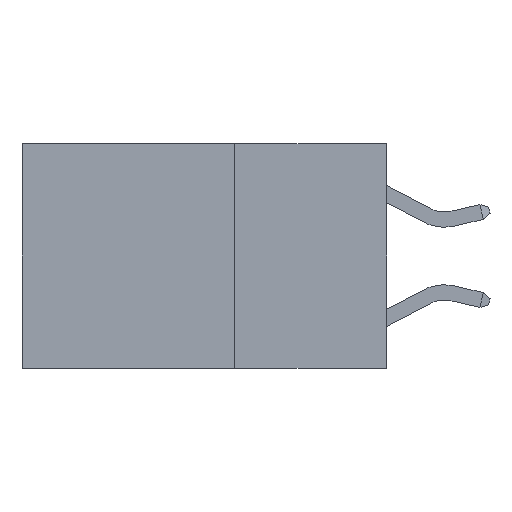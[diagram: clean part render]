
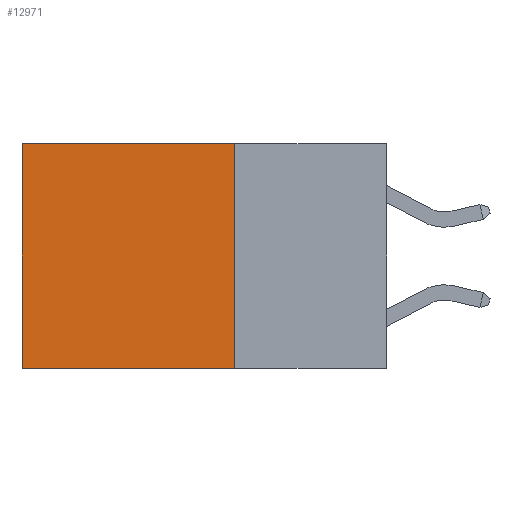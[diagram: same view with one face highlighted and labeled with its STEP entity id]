
A CAD part, left-side view. The second image highlights one B-rep face of the part: STEP entity #12971.
In plain terms, the highlighted planar face has unit normal (-1, 0, 0).
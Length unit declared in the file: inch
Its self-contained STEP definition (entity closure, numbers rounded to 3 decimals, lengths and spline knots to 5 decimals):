
#107 = VERTEX_POINT ( 'NONE', #5444 ) ;
#319 = PLANE ( 'NONE',  #3180 ) ;
#429 = CARTESIAN_POINT ( 'NONE',  ( 0.2625, 0.25, 0. ) ) ;
#506 = LINE ( 'NONE', #429, #14745 ) ;
#644 = DIRECTION ( 'NONE',  ( 0., 0., -1. ) ) ;
#1274 = VECTOR ( 'NONE', #12348, 39.37008 ) ;
#1816 = CARTESIAN_POINT ( 'NONE',  ( 0.2625, 0.6, -0.37 ) ) ;
#1836 = DIRECTION ( 'NONE',  ( 0., 0., -1. ) ) ;
#2252 = EDGE_LOOP ( 'NONE', ( #14381, #6729, #11589, #6524 ) ) ;
#3171 = EDGE_CURVE ( 'NONE', #15332, #3695, #506, .T. ) ;
#3180 = AXIS2_PLACEMENT_3D ( 'NONE', #10786, #8095, #644 ) ;
#3695 = VERTEX_POINT ( 'NONE', #15940 ) ;
#4331 = VECTOR ( 'NONE', #13352, 39.37008 ) ;
#5444 = CARTESIAN_POINT ( 'NONE',  ( 0.2625, 0.25, -0.37 ) ) ;
#5602 = VECTOR ( 'NONE', #1836, 39.37008 ) ;
#5854 = CARTESIAN_POINT ( 'NONE',  ( 0.2625, 0.25, -0.37 ) ) ;
#6524 = ORIENTED_EDGE ( 'NONE', *, *, #3171, .T. ) ;
#6729 = ORIENTED_EDGE ( 'NONE', *, *, #10629, .F. ) ;
#7406 = CARTESIAN_POINT ( 'NONE',  ( 0.2625, 0.6, 0. ) ) ;
#8095 = DIRECTION ( 'NONE',  ( 1., 0., 0. ) ) ;
#9372 = LINE ( 'NONE', #10867, #5602 ) ;
#10629 = EDGE_CURVE ( 'NONE', #107, #14761, #12261, .T. ) ;
#10786 = CARTESIAN_POINT ( 'NONE',  ( 0.2625, 0.25, 0. ) ) ;
#10867 = CARTESIAN_POINT ( 'NONE',  ( 0.2625, 0.25, 0. ) ) ;
#11589 = ORIENTED_EDGE ( 'NONE', *, *, #12950, .F. ) ;
#12261 = LINE ( 'NONE', #5854, #1274 ) ;
#12348 = DIRECTION ( 'NONE',  ( 0., 1., 0. ) ) ;
#12950 = EDGE_CURVE ( 'NONE', #15332, #107, #9372, .T. ) ;
#12971 = ADVANCED_FACE ( 'NONE', ( #13560 ), #319, .F. ) ;
#13352 = DIRECTION ( 'NONE',  ( 0., 0., -1. ) ) ;
#13560 = FACE_OUTER_BOUND ( 'NONE', #2252, .T. ) ;
#13649 = LINE ( 'NONE', #7406, #4331 ) ;
#14381 = ORIENTED_EDGE ( 'NONE', *, *, #15922, .T. ) ;
#14436 = DIRECTION ( 'NONE',  ( 0., 1., 0. ) ) ;
#14745 = VECTOR ( 'NONE', #14436, 39.37008 ) ;
#14761 = VERTEX_POINT ( 'NONE', #1816 ) ;
#15332 = VERTEX_POINT ( 'NONE', #16239 ) ;
#15922 = EDGE_CURVE ( 'NONE', #3695, #14761, #13649, .T. ) ;
#15940 = CARTESIAN_POINT ( 'NONE',  ( 0.2625, 0.6, 0. ) ) ;
#16239 = CARTESIAN_POINT ( 'NONE',  ( 0.2625, 0.25, 0. ) ) ;
